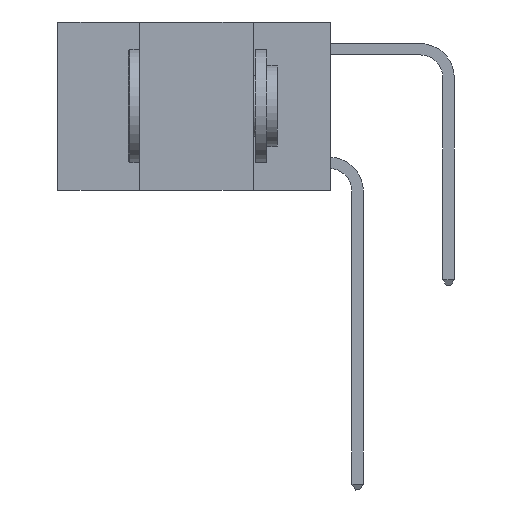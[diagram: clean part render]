
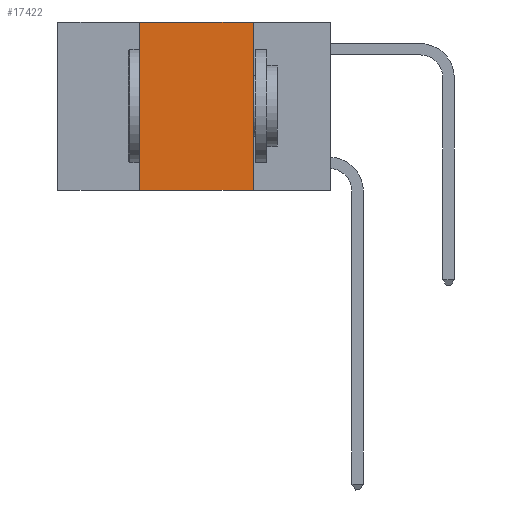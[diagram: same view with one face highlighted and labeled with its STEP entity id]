
A CAD part, left-side view. The second image highlights one B-rep face of the part: STEP entity #17422.
In plain terms, the highlighted planar face has unit normal (-1, 0, 0).
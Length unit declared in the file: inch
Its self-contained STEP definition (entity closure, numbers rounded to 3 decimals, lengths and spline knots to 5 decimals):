
#213 = LINE ( 'NONE', #16844, #10297 ) ;
#217 = VERTEX_POINT ( 'NONE', #1552 ) ;
#481 = VERTEX_POINT ( 'NONE', #15062 ) ;
#1083 = CARTESIAN_POINT ( 'NONE',  ( 0., 0.17, 0. ) ) ;
#1552 = CARTESIAN_POINT ( 'NONE',  ( 0., 0.42, -0.37 ) ) ;
#2973 = PLANE ( 'NONE',  #5354 ) ;
#3885 = DIRECTION ( 'NONE',  ( 0., 0., 1. ) ) ;
#4041 = ORIENTED_EDGE ( 'NONE', *, *, #9579, .F. ) ;
#4576 = DIRECTION ( 'NONE',  ( 0., -1., 0. ) ) ;
#5354 = AXIS2_PLACEMENT_3D ( 'NONE', #13035, #5627, #13220 ) ;
#5627 = DIRECTION ( 'NONE',  ( 1., 0., 0. ) ) ;
#7316 = EDGE_CURVE ( 'NONE', #217, #9407, #10099, .T. ) ;
#7367 = VECTOR ( 'NONE', #10684, 39.37008 ) ;
#7418 = FACE_OUTER_BOUND ( 'NONE', #16979, .T. ) ;
#9407 = VERTEX_POINT ( 'NONE', #12445 ) ;
#9579 = EDGE_CURVE ( 'NONE', #481, #9974, #16110, .T. ) ;
#9974 = VERTEX_POINT ( 'NONE', #11516 ) ;
#10099 = LINE ( 'NONE', #19307, #13187 ) ;
#10297 = VECTOR ( 'NONE', #4576, 39.37008 ) ;
#10684 = DIRECTION ( 'NONE',  ( 0., -1., 0. ) ) ;
#11516 = CARTESIAN_POINT ( 'NONE',  ( 0., 0.17, -0.37 ) ) ;
#11782 = ORIENTED_EDGE ( 'NONE', *, *, #17237, .F. ) ;
#12037 = ORIENTED_EDGE ( 'NONE', *, *, #14448, .T. ) ;
#12317 = VECTOR ( 'NONE', #17685, 39.37008 ) ;
#12445 = CARTESIAN_POINT ( 'NONE',  ( 0., 0.42, 0. ) ) ;
#13035 = CARTESIAN_POINT ( 'NONE',  ( 0., 0.6, 0. ) ) ;
#13187 = VECTOR ( 'NONE', #3885, 39.37008 ) ;
#13220 = DIRECTION ( 'NONE',  ( 0., 0., -1. ) ) ;
#13538 = CARTESIAN_POINT ( 'NONE',  ( 0., 0.6, -0.37 ) ) ;
#14448 = EDGE_CURVE ( 'NONE', #217, #9974, #18311, .T. ) ;
#14727 = ORIENTED_EDGE ( 'NONE', *, *, #7316, .F. ) ;
#15062 = CARTESIAN_POINT ( 'NONE',  ( 0., 0.17, 0. ) ) ;
#16110 = LINE ( 'NONE', #1083, #12317 ) ;
#16844 = CARTESIAN_POINT ( 'NONE',  ( 0., 0.6, 0. ) ) ;
#16979 = EDGE_LOOP ( 'NONE', ( #4041, #11782, #14727, #12037 ) ) ;
#17237 = EDGE_CURVE ( 'NONE', #9407, #481, #213, .T. ) ;
#17422 = ADVANCED_FACE ( 'NONE', ( #7418 ), #2973, .F. ) ;
#17685 = DIRECTION ( 'NONE',  ( 0., 0., -1. ) ) ;
#18311 = LINE ( 'NONE', #13538, #7367 ) ;
#19307 = CARTESIAN_POINT ( 'NONE',  ( 0., 0.42, 0. ) ) ;
